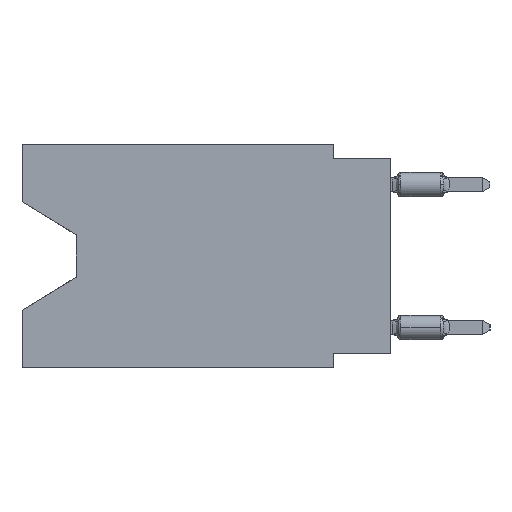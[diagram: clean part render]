
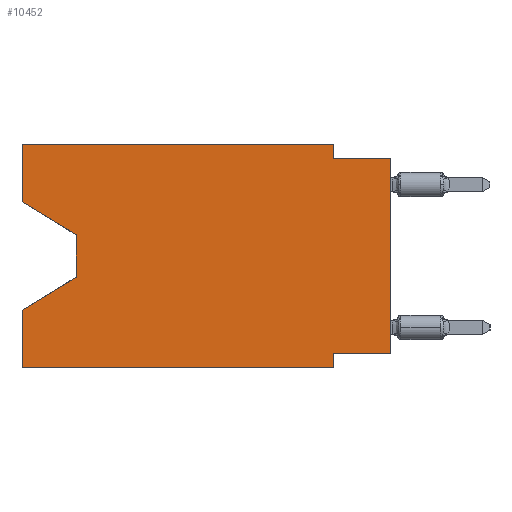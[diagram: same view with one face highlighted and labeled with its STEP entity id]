
A CAD part, left-side view. The second image highlights one B-rep face of the part: STEP entity #10452.
In plain terms, the highlighted planar face has unit normal (-1, 0, 0).
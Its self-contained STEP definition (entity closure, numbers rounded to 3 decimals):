
#600 = ORIENTED_EDGE ( 'NONE', *, *, #3916, .T. ) ;
#780 = ORIENTED_EDGE ( 'NONE', *, *, #19833, .T. ) ;
#1285 = CARTESIAN_POINT ( 'NONE',  ( 0., 16.383, 0. ) ) ;
#1581 = CARTESIAN_POINT ( 'NONE',  ( 0., 16.383, 0. ) ) ;
#1741 = CARTESIAN_POINT ( 'NONE',  ( 0., 16.383, 0. ) ) ;
#1842 = LINE ( 'NONE', #18651, #26934 ) ;
#1987 = DIRECTION ( 'NONE',  ( 0., 0., 1. ) ) ;
#2613 = LINE ( 'NONE', #5002, #14096 ) ;
#2851 = VERTEX_POINT ( 'NONE', #30013 ) ;
#2867 = VERTEX_POINT ( 'NONE', #1581 ) ;
#2868 = VECTOR ( 'NONE', #11437, 1000. ) ;
#2911 = EDGE_CURVE ( 'NONE', #2867, #2851, #26192, .T. ) ;
#3529 = VERTEX_POINT ( 'NONE', #27085 ) ;
#3761 = EDGE_CURVE ( 'NONE', #5898, #14487, #19114, .T. ) ;
#3916 = EDGE_CURVE ( 'NONE', #27527, #14487, #2613, .T. ) ;
#3938 = LINE ( 'NONE', #30768, #7761 ) ;
#4175 = LINE ( 'NONE', #20985, #14344 ) ;
#4310 = VECTOR ( 'NONE', #24695, 1000. ) ;
#4539 = CARTESIAN_POINT ( 'NONE',  ( 0., 16.383, 0. ) ) ;
#5002 = CARTESIAN_POINT ( 'NONE',  ( 0., 13.97, -5.893 ) ) ;
#5898 = VERTEX_POINT ( 'NONE', #22057 ) ;
#6864 = CARTESIAN_POINT ( 'NONE',  ( 0., 0., -0.635 ) ) ;
#6937 = ORIENTED_EDGE ( 'NONE', *, *, #2911, .F. ) ;
#7442 = DIRECTION ( 'NONE',  ( 0., -1., 0. ) ) ;
#7761 = VECTOR ( 'NONE', #16609, 1000. ) ;
#8175 = EDGE_CURVE ( 'NONE', #29619, #27527, #9039, .T. ) ;
#8755 = PLANE ( 'NONE',  #16287 ) ;
#8955 = LINE ( 'NONE', #9113, #17967 ) ;
#9039 = LINE ( 'NONE', #25544, #19712 ) ;
#9113 = CARTESIAN_POINT ( 'NONE',  ( 0., 16.383, -2.546 ) ) ;
#9644 = EDGE_CURVE ( 'NONE', #14962, #2867, #19372, .T. ) ;
#9811 = LINE ( 'NONE', #29187, #23870 ) ;
#10452 = ADVANCED_FACE ( 'NONE', ( #23031 ), #8755, .F. ) ;
#11437 = DIRECTION ( 'NONE',  ( 0., -1., 0. ) ) ;
#12621 = CARTESIAN_POINT ( 'NONE',  ( 0., 2.54, -0.635 ) ) ;
#12629 = VERTEX_POINT ( 'NONE', #27247 ) ;
#12708 = CARTESIAN_POINT ( 'NONE',  ( 0., 13.97, -4.013 ) ) ;
#12792 = ORIENTED_EDGE ( 'NONE', *, *, #15643, .T. ) ;
#12960 = CARTESIAN_POINT ( 'NONE',  ( 0., 16.383, -2.546 ) ) ;
#13511 = DIRECTION ( 'NONE',  ( 0., 0., -1. ) ) ;
#13774 = DIRECTION ( 'NONE',  ( 0., 1., 0. ) ) ;
#13931 = EDGE_CURVE ( 'NONE', #12629, #3529, #1842, .T. ) ;
#13970 = CARTESIAN_POINT ( 'NONE',  ( 0., 0., -9.271 ) ) ;
#14096 = VECTOR ( 'NONE', #14668, 1000. ) ;
#14112 = ORIENTED_EDGE ( 'NONE', *, *, #3761, .F. ) ;
#14333 = DIRECTION ( 'NONE',  ( 0., -0.855, -0.519 ) ) ;
#14344 = VECTOR ( 'NONE', #30049, 1000. ) ;
#14487 = VERTEX_POINT ( 'NONE', #31333 ) ;
#14668 = DIRECTION ( 'NONE',  ( 0., 0.855, -0.519 ) ) ;
#14689 = EDGE_CURVE ( 'NONE', #24195, #12629, #20760, .T. ) ;
#14852 = LINE ( 'NONE', #15002, #4310 ) ;
#14962 = VERTEX_POINT ( 'NONE', #12960 ) ;
#14969 = EDGE_CURVE ( 'NONE', #5898, #3529, #9811, .T. ) ;
#15002 = CARTESIAN_POINT ( 'NONE',  ( 0., 0., -0.635 ) ) ;
#15643 = EDGE_CURVE ( 'NONE', #14962, #29619, #8955, .T. ) ;
#15947 = ORIENTED_EDGE ( 'NONE', *, *, #8175, .T. ) ;
#15949 = DIRECTION ( 'NONE',  ( 0., 0., -1. ) ) ;
#16184 = DIRECTION ( 'NONE',  ( 1., 0., 0. ) ) ;
#16287 = AXIS2_PLACEMENT_3D ( 'NONE', #1285, #16184, #13511 ) ;
#16435 = EDGE_LOOP ( 'NONE', ( #12792, #15947, #600, #14112, #26294, #25189, #24613, #780, #26904, #23404, #6937, #24677 ) ) ;
#16609 = DIRECTION ( 'NONE',  ( 0., 0., 1. ) ) ;
#16641 = VERTEX_POINT ( 'NONE', #12621 ) ;
#16987 = CARTESIAN_POINT ( 'NONE',  ( 0., 16.383, 0. ) ) ;
#17683 = CARTESIAN_POINT ( 'NONE',  ( 0., 13.97, -5.893 ) ) ;
#17967 = VECTOR ( 'NONE', #14333, 1000. ) ;
#18651 = CARTESIAN_POINT ( 'NONE',  ( 0., 2.54, -9.906 ) ) ;
#19114 = LINE ( 'NONE', #4539, #27755 ) ;
#19372 = LINE ( 'NONE', #16987, #23444 ) ;
#19476 = EDGE_CURVE ( 'NONE', #2851, #16641, #4175, .T. ) ;
#19712 = VECTOR ( 'NONE', #25382, 1000. ) ;
#19833 = EDGE_CURVE ( 'NONE', #24195, #29460, #3938, .T. ) ;
#20760 = LINE ( 'NONE', #22991, #26976 ) ;
#20985 = CARTESIAN_POINT ( 'NONE',  ( 0., 2.54, 0. ) ) ;
#22057 = CARTESIAN_POINT ( 'NONE',  ( 0., 16.383, -9.906 ) ) ;
#22991 = CARTESIAN_POINT ( 'NONE',  ( 0., 0., -9.271 ) ) ;
#23031 = FACE_OUTER_BOUND ( 'NONE', #16435, .T. ) ;
#23404 = ORIENTED_EDGE ( 'NONE', *, *, #19476, .F. ) ;
#23444 = VECTOR ( 'NONE', #24146, 1000. ) ;
#23870 = VECTOR ( 'NONE', #7442, 1000. ) ;
#24146 = DIRECTION ( 'NONE',  ( 0., 0., 1. ) ) ;
#24195 = VERTEX_POINT ( 'NONE', #13970 ) ;
#24613 = ORIENTED_EDGE ( 'NONE', *, *, #14689, .F. ) ;
#24677 = ORIENTED_EDGE ( 'NONE', *, *, #9644, .F. ) ;
#24695 = DIRECTION ( 'NONE',  ( 0., -1., 0. ) ) ;
#25189 = ORIENTED_EDGE ( 'NONE', *, *, #13931, .F. ) ;
#25382 = DIRECTION ( 'NONE',  ( 0., 0., -1. ) ) ;
#25544 = CARTESIAN_POINT ( 'NONE',  ( 0., 13.97, -4.013 ) ) ;
#26192 = LINE ( 'NONE', #1741, #2868 ) ;
#26294 = ORIENTED_EDGE ( 'NONE', *, *, #14969, .T. ) ;
#26904 = ORIENTED_EDGE ( 'NONE', *, *, #27634, .F. ) ;
#26934 = VECTOR ( 'NONE', #15949, 1000. ) ;
#26976 = VECTOR ( 'NONE', #13774, 1000. ) ;
#27085 = CARTESIAN_POINT ( 'NONE',  ( 0., 2.54, -9.906 ) ) ;
#27247 = CARTESIAN_POINT ( 'NONE',  ( 0., 2.54, -9.271 ) ) ;
#27527 = VERTEX_POINT ( 'NONE', #17683 ) ;
#27634 = EDGE_CURVE ( 'NONE', #16641, #29460, #14852, .T. ) ;
#27755 = VECTOR ( 'NONE', #1987, 1000. ) ;
#29187 = CARTESIAN_POINT ( 'NONE',  ( 0., 16.383, -9.906 ) ) ;
#29460 = VERTEX_POINT ( 'NONE', #6864 ) ;
#29619 = VERTEX_POINT ( 'NONE', #12708 ) ;
#30013 = CARTESIAN_POINT ( 'NONE',  ( 0., 2.54, 0. ) ) ;
#30049 = DIRECTION ( 'NONE',  ( 0., 0., -1. ) ) ;
#30768 = CARTESIAN_POINT ( 'NONE',  ( 0., 0., 0. ) ) ;
#31333 = CARTESIAN_POINT ( 'NONE',  ( 0., 16.383, -7.36 ) ) ;
